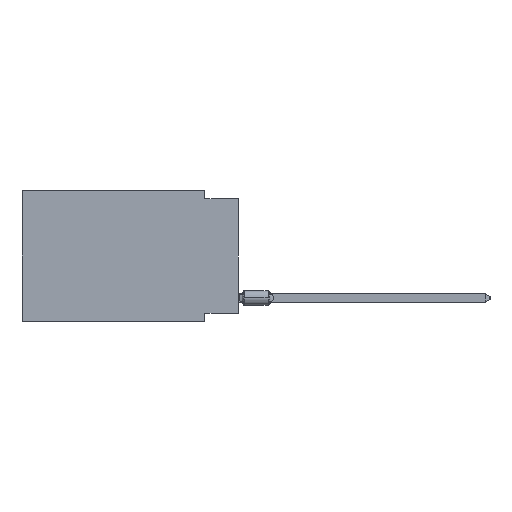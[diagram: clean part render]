
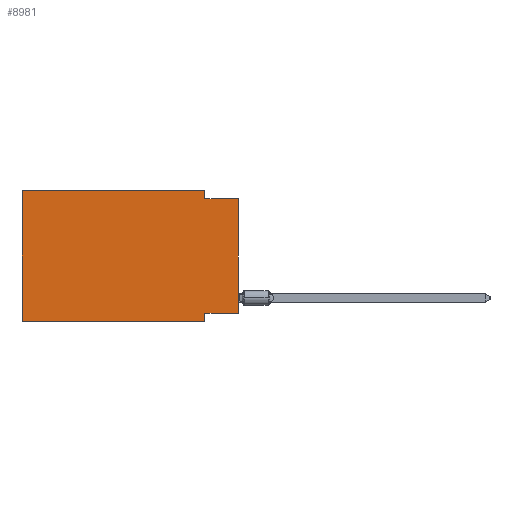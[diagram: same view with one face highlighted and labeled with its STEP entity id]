
A CAD part, left-side view. The second image highlights one B-rep face of the part: STEP entity #8981.
In plain terms, the highlighted planar face has unit normal (-1, 0, 0).
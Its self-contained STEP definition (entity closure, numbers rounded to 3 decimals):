
#1425 = ORIENTED_EDGE ( 'NONE', *, *, #57054, .F. ) ;
#1843 = CARTESIAN_POINT ( 'NONE',  ( 0., 16.383, 0. ) ) ;
#2978 = EDGE_CURVE ( 'NONE', #19501, #33281, #27127, .T. ) ;
#3052 = EDGE_LOOP ( 'NONE', ( #55108, #66870, #41409, #7682, #63197, #69578, #1425, #14342 ) ) ;
#4321 = CARTESIAN_POINT ( 'NONE',  ( 0., 0., -0.635 ) ) ;
#6618 = VERTEX_POINT ( 'NONE', #61523 ) ;
#7682 = ORIENTED_EDGE ( 'NONE', *, *, #38013, .F. ) ;
#8981 = ADVANCED_FACE ( 'NONE', ( #69252 ), #52210, .F. ) ;
#9960 = LINE ( 'NONE', #15059, #56397 ) ;
#10377 = CARTESIAN_POINT ( 'NONE',  ( 0., 0., -9.271 ) ) ;
#10438 = VECTOR ( 'NONE', #64306, 1000. ) ;
#10447 = DIRECTION ( 'NONE',  ( 0., 0., 1. ) ) ;
#10813 = VECTOR ( 'NONE', #20579, 1000. ) ;
#11446 = CARTESIAN_POINT ( 'NONE',  ( 0., 16.383, 0. ) ) ;
#14342 = ORIENTED_EDGE ( 'NONE', *, *, #71366, .F. ) ;
#15059 = CARTESIAN_POINT ( 'NONE',  ( 0., 0., -9.271 ) ) ;
#15486 = LINE ( 'NONE', #15849, #21036 ) ;
#15849 = CARTESIAN_POINT ( 'NONE',  ( 0., 2.54, -9.906 ) ) ;
#16950 = VERTEX_POINT ( 'NONE', #35920 ) ;
#16984 = CARTESIAN_POINT ( 'NONE',  ( 0., 2.54, 0. ) ) ;
#18054 = CARTESIAN_POINT ( 'NONE',  ( 0., 16.383, -9.906 ) ) ;
#18882 = VECTOR ( 'NONE', #10447, 1000. ) ;
#19501 = VERTEX_POINT ( 'NONE', #55011 ) ;
#20053 = LINE ( 'NONE', #26557, #10438 ) ;
#20579 = DIRECTION ( 'NONE',  ( 0., -1., 0. ) ) ;
#20958 = CARTESIAN_POINT ( 'NONE',  ( 0., 16.383, 0. ) ) ;
#21036 = VECTOR ( 'NONE', #25993, 1000. ) ;
#22335 = EDGE_CURVE ( 'NONE', #45228, #46192, #54540, .T. ) ;
#23929 = DIRECTION ( 'NONE',  ( 1., 0., 0. ) ) ;
#25993 = DIRECTION ( 'NONE',  ( 0., 0., -1. ) ) ;
#26557 = CARTESIAN_POINT ( 'NONE',  ( 0., 0., -0.635 ) ) ;
#27127 = LINE ( 'NONE', #20958, #18882 ) ;
#27312 = DIRECTION ( 'NONE',  ( 0., 0., 1. ) ) ;
#33265 = VERTEX_POINT ( 'NONE', #49180 ) ;
#33281 = VERTEX_POINT ( 'NONE', #11446 ) ;
#34032 = LINE ( 'NONE', #18054, #56988 ) ;
#35920 = CARTESIAN_POINT ( 'NONE',  ( 0., 2.54, -9.271 ) ) ;
#37180 = DIRECTION ( 'NONE',  ( 0., 1., 0. ) ) ;
#38013 = EDGE_CURVE ( 'NONE', #33281, #33265, #53602, .T. ) ;
#39632 = CARTESIAN_POINT ( 'NONE',  ( 0., 0., 0. ) ) ;
#40000 = EDGE_CURVE ( 'NONE', #6618, #46192, #20053, .T. ) ;
#40054 = VECTOR ( 'NONE', #27312, 1000. ) ;
#41409 = ORIENTED_EDGE ( 'NONE', *, *, #50530, .F. ) ;
#43822 = EDGE_CURVE ( 'NONE', #19501, #67427, #34032, .T. ) ;
#43839 = DIRECTION ( 'NONE',  ( 0., 0., -1. ) ) ;
#45228 = VERTEX_POINT ( 'NONE', #10377 ) ;
#46192 = VERTEX_POINT ( 'NONE', #4321 ) ;
#46770 = DIRECTION ( 'NONE',  ( 0., 0., -1. ) ) ;
#49180 = CARTESIAN_POINT ( 'NONE',  ( 0., 2.54, 0. ) ) ;
#50530 = EDGE_CURVE ( 'NONE', #33265, #6618, #55433, .T. ) ;
#52210 = PLANE ( 'NONE',  #62262 ) ;
#53602 = LINE ( 'NONE', #69928, #10813 ) ;
#54540 = LINE ( 'NONE', #39632, #40054 ) ;
#55011 = CARTESIAN_POINT ( 'NONE',  ( 0., 16.383, -9.906 ) ) ;
#55108 = ORIENTED_EDGE ( 'NONE', *, *, #22335, .T. ) ;
#55433 = LINE ( 'NONE', #16984, #69272 ) ;
#56397 = VECTOR ( 'NONE', #37180, 1000. ) ;
#56988 = VECTOR ( 'NONE', #57936, 1000. ) ;
#57054 = EDGE_CURVE ( 'NONE', #16950, #67427, #15486, .T. ) ;
#57936 = DIRECTION ( 'NONE',  ( 0., -1., 0. ) ) ;
#61523 = CARTESIAN_POINT ( 'NONE',  ( 0., 2.54, -0.635 ) ) ;
#62262 = AXIS2_PLACEMENT_3D ( 'NONE', #1843, #23929, #46770 ) ;
#63197 = ORIENTED_EDGE ( 'NONE', *, *, #2978, .F. ) ;
#64306 = DIRECTION ( 'NONE',  ( 0., -1., 0. ) ) ;
#66174 = CARTESIAN_POINT ( 'NONE',  ( 0., 2.54, -9.906 ) ) ;
#66870 = ORIENTED_EDGE ( 'NONE', *, *, #40000, .F. ) ;
#67427 = VERTEX_POINT ( 'NONE', #66174 ) ;
#69252 = FACE_OUTER_BOUND ( 'NONE', #3052, .T. ) ;
#69272 = VECTOR ( 'NONE', #43839, 1000. ) ;
#69578 = ORIENTED_EDGE ( 'NONE', *, *, #43822, .T. ) ;
#69928 = CARTESIAN_POINT ( 'NONE',  ( 0., 16.383, 0. ) ) ;
#71366 = EDGE_CURVE ( 'NONE', #45228, #16950, #9960, .T. ) ;
